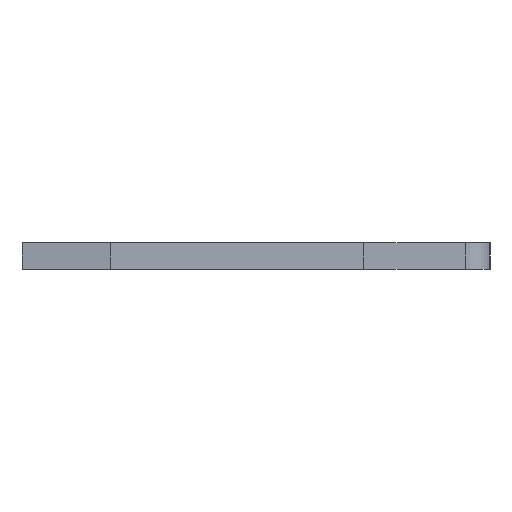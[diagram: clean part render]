
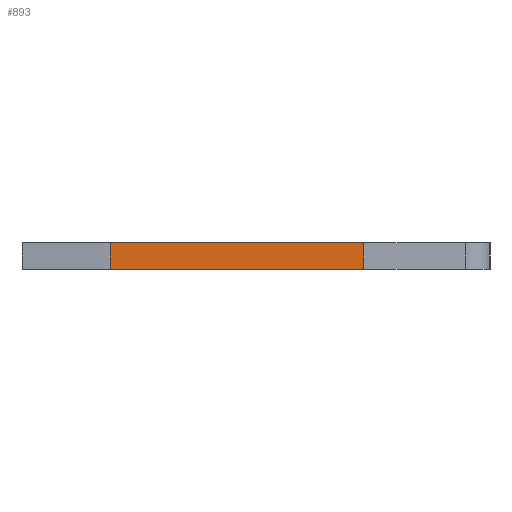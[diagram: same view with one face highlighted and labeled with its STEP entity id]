
A CAD part, left-side view. The second image highlights one B-rep face of the part: STEP entity #893.
In plain terms, the highlighted face is planar.
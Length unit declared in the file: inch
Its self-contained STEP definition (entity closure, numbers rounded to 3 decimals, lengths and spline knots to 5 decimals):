
#15 = DIRECTION ( 'NONE',  ( 0., 1., 0. ) ) ;
#44 = DIRECTION ( 'NONE',  ( -1., 0., 0. ) ) ;
#57 = CARTESIAN_POINT ( 'NONE',  ( -0.013, 0.146, -0.0575 ) ) ;
#58 = VERTEX_POINT ( 'NONE', #1251 ) ;
#94 = CARTESIAN_POINT ( 'NONE',  ( 0.013, -0.099, -0.0575 ) ) ;
#112 = ORIENTED_EDGE ( 'NONE', *, *, #804, .F. ) ;
#131 = VERTEX_POINT ( 'NONE', #1549 ) ;
#203 = EDGE_CURVE ( 'NONE', #1321, #1612, #1658, .T. ) ;
#249 = FACE_OUTER_BOUND ( 'NONE', #639, .T. ) ;
#320 = VECTOR ( 'NONE', #44, 39.37008 ) ;
#501 = DIRECTION ( 'NONE',  ( -1., 0., 0. ) ) ;
#553 = VECTOR ( 'NONE', #1371, 39.37008 ) ;
#625 = CARTESIAN_POINT ( 'NONE',  ( 0.013, 0.146, -0.0575 ) ) ;
#636 = VECTOR ( 'NONE', #501, 39.37008 ) ;
#639 = EDGE_LOOP ( 'NONE', ( #1813, #112, #1195, #1362 ) ) ;
#642 = EDGE_CURVE ( 'NONE', #1321, #58, #1683, .T. ) ;
#749 = CARTESIAN_POINT ( 'NONE',  ( 0.013, -0.099, -0.0575 ) ) ;
#804 = EDGE_CURVE ( 'NONE', #1612, #131, #965, .T. ) ;
#893 = ADVANCED_FACE ( 'NONE', ( #249 ), #1505, .F. ) ;
#911 = EDGE_CURVE ( 'NONE', #58, #131, #1314, .T. ) ;
#965 = LINE ( 'NONE', #1067, #636 ) ;
#1067 = CARTESIAN_POINT ( 'NONE',  ( 0.013, 0.146, -0.0575 ) ) ;
#1191 = VECTOR ( 'NONE', #15, 39.37008 ) ;
#1195 = ORIENTED_EDGE ( 'NONE', *, *, #203, .F. ) ;
#1223 = DIRECTION ( 'NONE',  ( 0., 0., 1. ) ) ;
#1251 = CARTESIAN_POINT ( 'NONE',  ( -0.013, -0.099, -0.0575 ) ) ;
#1314 = LINE ( 'NONE', #57, #553 ) ;
#1321 = VERTEX_POINT ( 'NONE', #94 ) ;
#1354 = DIRECTION ( 'NONE',  ( 1., 0., 0. ) ) ;
#1362 = ORIENTED_EDGE ( 'NONE', *, *, #642, .T. ) ;
#1371 = DIRECTION ( 'NONE',  ( 0., 1., 0. ) ) ;
#1425 = CARTESIAN_POINT ( 'NONE',  ( 0.013, 0.146, -0.0575 ) ) ;
#1505 = PLANE ( 'NONE',  #1723 ) ;
#1549 = CARTESIAN_POINT ( 'NONE',  ( -0.013, 0.146, -0.0575 ) ) ;
#1612 = VERTEX_POINT ( 'NONE', #1425 ) ;
#1658 = LINE ( 'NONE', #1699, #1191 ) ;
#1683 = LINE ( 'NONE', #749, #320 ) ;
#1699 = CARTESIAN_POINT ( 'NONE',  ( 0.013, 0.146, -0.0575 ) ) ;
#1723 = AXIS2_PLACEMENT_3D ( 'NONE', #625, #1223, #1354 ) ;
#1813 = ORIENTED_EDGE ( 'NONE', *, *, #911, .T. ) ;
